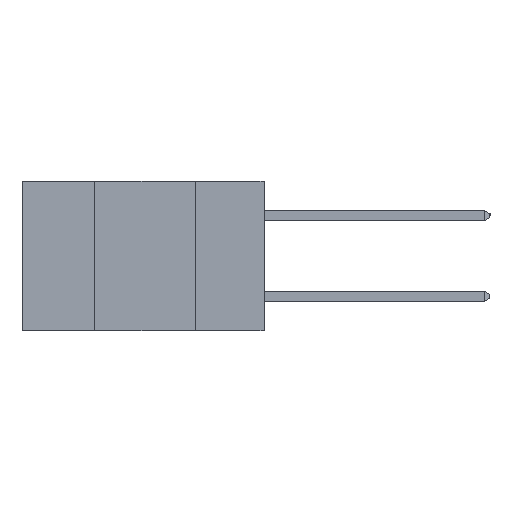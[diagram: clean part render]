
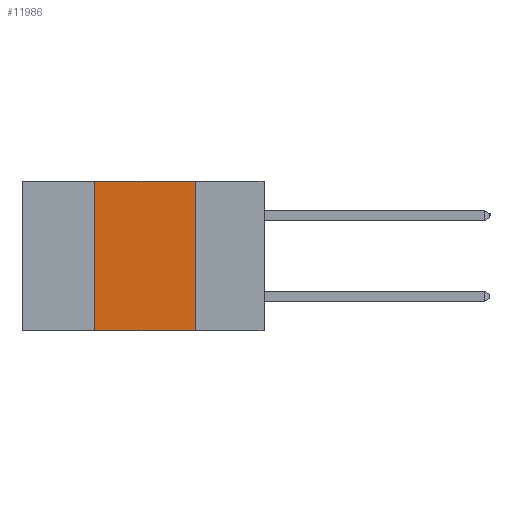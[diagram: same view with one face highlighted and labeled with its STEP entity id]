
A CAD part, left-side view. The second image highlights one B-rep face of the part: STEP entity #11986.
In plain terms, the highlighted planar face has unit normal (-1, 0, 0).
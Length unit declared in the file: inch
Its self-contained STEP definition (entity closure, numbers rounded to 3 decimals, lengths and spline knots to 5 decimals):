
#743 = CARTESIAN_POINT ( 'NONE',  ( 0., 0.17, 0. ) ) ;
#1922 = CARTESIAN_POINT ( 'NONE',  ( 0., 0.42, -0.37 ) ) ;
#2225 = EDGE_CURVE ( 'NONE', #4508, #8751, #9166, .T. ) ;
#2237 = EDGE_LOOP ( 'NONE', ( #7583, #3968, #9037, #3196 ) ) ;
#2563 = VECTOR ( 'NONE', #12617, 39.37008 ) ;
#2660 = DIRECTION ( 'NONE',  ( 1., 0., 0. ) ) ;
#3196 = ORIENTED_EDGE ( 'NONE', *, *, #8003, .T. ) ;
#3341 = DIRECTION ( 'NONE',  ( 0., -1., 0. ) ) ;
#3579 = DIRECTION ( 'NONE',  ( 0., 0., -1. ) ) ;
#3822 = CARTESIAN_POINT ( 'NONE',  ( 0., 0.6, 0. ) ) ;
#3968 = ORIENTED_EDGE ( 'NONE', *, *, #2225, .F. ) ;
#4508 = VERTEX_POINT ( 'NONE', #7919 ) ;
#5526 = LINE ( 'NONE', #6608, #11258 ) ;
#5733 = EDGE_CURVE ( 'NONE', #8751, #8822, #8825, .T. ) ;
#5797 = DIRECTION ( 'NONE',  ( 0., 0., -1. ) ) ;
#5872 = FACE_OUTER_BOUND ( 'NONE', #2237, .T. ) ;
#6608 = CARTESIAN_POINT ( 'NONE',  ( 0., 0.6, -0.37 ) ) ;
#6879 = PLANE ( 'NONE',  #11133 ) ;
#7583 = ORIENTED_EDGE ( 'NONE', *, *, #5733, .F. ) ;
#7674 = CARTESIAN_POINT ( 'NONE',  ( 0., 0.17, -0.37 ) ) ;
#7919 = CARTESIAN_POINT ( 'NONE',  ( 0., 0.42, 0. ) ) ;
#8003 = EDGE_CURVE ( 'NONE', #11498, #8822, #5526, .T. ) ;
#8207 = CARTESIAN_POINT ( 'NONE',  ( 0., 0.6, 0. ) ) ;
#8400 = EDGE_CURVE ( 'NONE', #11498, #4508, #11599, .T. ) ;
#8449 = CARTESIAN_POINT ( 'NONE',  ( 0., 0.17, -0.37 ) ) ;
#8751 = VERTEX_POINT ( 'NONE', #743 ) ;
#8822 = VERTEX_POINT ( 'NONE', #8449 ) ;
#8825 = LINE ( 'NONE', #7674, #9750 ) ;
#9037 = ORIENTED_EDGE ( 'NONE', *, *, #8400, .F. ) ;
#9166 = LINE ( 'NONE', #8207, #11488 ) ;
#9750 = VECTOR ( 'NONE', #3579, 39.37008 ) ;
#10656 = CARTESIAN_POINT ( 'NONE',  ( 0., 0.42, -0.37 ) ) ;
#11133 = AXIS2_PLACEMENT_3D ( 'NONE', #3822, #2660, #5797 ) ;
#11258 = VECTOR ( 'NONE', #3341, 39.37008 ) ;
#11488 = VECTOR ( 'NONE', #13325, 39.37008 ) ;
#11498 = VERTEX_POINT ( 'NONE', #1922 ) ;
#11599 = LINE ( 'NONE', #10656, #2563 ) ;
#11986 = ADVANCED_FACE ( 'NONE', ( #5872 ), #6879, .F. ) ;
#12617 = DIRECTION ( 'NONE',  ( 0., 0., 1. ) ) ;
#13325 = DIRECTION ( 'NONE',  ( 0., -1., 0. ) ) ;
